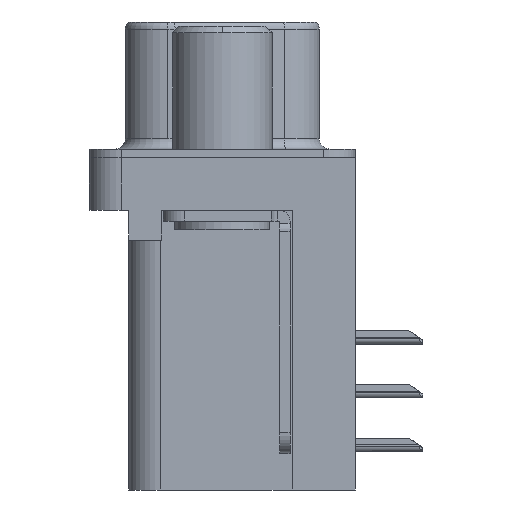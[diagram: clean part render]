
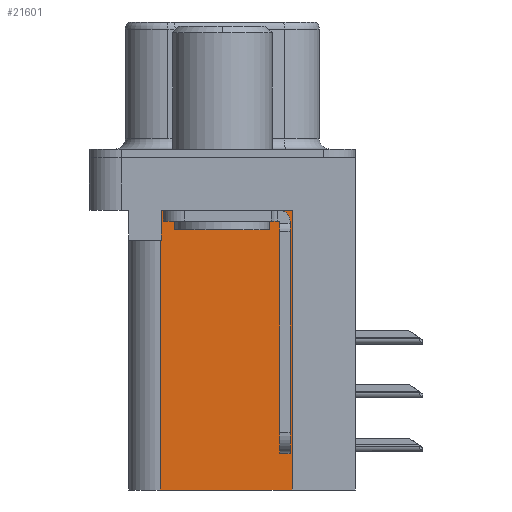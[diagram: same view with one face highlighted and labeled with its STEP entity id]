
A CAD part, left-side view. The second image highlights one B-rep face of the part: STEP entity #21601.
In plain terms, the highlighted planar face has unit normal (-1, 0, 0).
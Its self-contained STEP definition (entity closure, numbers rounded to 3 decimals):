
#147 = LINE ( 'NONE', #256, #7849 ) ;
#256 = CARTESIAN_POINT ( 'NONE',  ( 3.79, -3.295, -2.5 ) ) ;
#668 = EDGE_CURVE ( 'NONE', #18045, #21970, #11261, .T. ) ;
#2689 = VECTOR ( 'NONE', #6367, 1000. ) ;
#3335 = CARTESIAN_POINT ( 'NONE',  ( 3.79, -3.295, -2.5 ) ) ;
#3836 = EDGE_CURVE ( 'NONE', #22131, #28776, #23106, .T. ) ;
#4481 = PLANE ( 'NONE',  #26786 ) ;
#4844 = ORIENTED_EDGE ( 'NONE', *, *, #17191, .T. ) ;
#4858 = VECTOR ( 'NONE', #14583, 1000. ) ;
#5062 = ORIENTED_EDGE ( 'NONE', *, *, #3836, .T. ) ;
#6367 = DIRECTION ( 'NONE',  ( 0., 0., -1. ) ) ;
#6426 = LINE ( 'NONE', #26292, #26932 ) ;
#6596 = EDGE_LOOP ( 'NONE', ( #20667, #27789, #5062, #28978, #11658, #4844 ) ) ;
#7565 = CARTESIAN_POINT ( 'NONE',  ( 3.79, 0., -3.9 ) ) ;
#7719 = VECTOR ( 'NONE', #26728, 1000. ) ;
#7849 = VECTOR ( 'NONE', #13999, 1000. ) ;
#11261 = LINE ( 'NONE', #20682, #4858 ) ;
#11658 = ORIENTED_EDGE ( 'NONE', *, *, #668, .F. ) ;
#12693 = VERTEX_POINT ( 'NONE', #3335 ) ;
#13999 = DIRECTION ( 'NONE',  ( 0., 1., 0. ) ) ;
#14583 = DIRECTION ( 'NONE',  ( 0., 1., 0. ) ) ;
#16010 = CARTESIAN_POINT ( 'NONE',  ( 3.79, 2.925, -15.7 ) ) ;
#17191 = EDGE_CURVE ( 'NONE', #18045, #12693, #6426, .T. ) ;
#17584 = CARTESIAN_POINT ( 'NONE',  ( 3.79, -3.295, -15.7 ) ) ;
#18045 = VERTEX_POINT ( 'NONE', #17584 ) ;
#18079 = DIRECTION ( 'NONE',  ( 0., 1., 0. ) ) ;
#18216 = DIRECTION ( 'NONE',  ( 0., 0., 1. ) ) ;
#18395 = CARTESIAN_POINT ( 'NONE',  ( 3.79, 2.895, -2.5 ) ) ;
#18473 = EDGE_CURVE ( 'NONE', #21970, #28776, #21713, .T. ) ;
#20667 = ORIENTED_EDGE ( 'NONE', *, *, #28998, .T. ) ;
#20682 = CARTESIAN_POINT ( 'NONE',  ( 3.79, -3.295, -15.7 ) ) ;
#21601 = ADVANCED_FACE ( 'NONE', ( #33226 ), #4481, .F. ) ;
#21713 = LINE ( 'NONE', #16010, #7719 ) ;
#21970 = VERTEX_POINT ( 'NONE', #33004 ) ;
#22131 = VERTEX_POINT ( 'NONE', #33439 ) ;
#22289 = CARTESIAN_POINT ( 'NONE',  ( 3.79, 2.895, -3.9 ) ) ;
#23106 = LINE ( 'NONE', #7565, #29615 ) ;
#23205 = CARTESIAN_POINT ( 'NONE',  ( 3.79, -3.295, -15.7 ) ) ;
#25995 = DIRECTION ( 'NONE',  ( 0., 0., -1. ) ) ;
#26219 = CARTESIAN_POINT ( 'NONE',  ( 3.79, 2.925, -3.9 ) ) ;
#26292 = CARTESIAN_POINT ( 'NONE',  ( 3.79, -3.295, -15.7 ) ) ;
#26728 = DIRECTION ( 'NONE',  ( 0., 0., 1. ) ) ;
#26786 = AXIS2_PLACEMENT_3D ( 'NONE', #23205, #34196, #25995 ) ;
#26932 = VECTOR ( 'NONE', #18216, 1000. ) ;
#27789 = ORIENTED_EDGE ( 'NONE', *, *, #34431, .T. ) ;
#28776 = VERTEX_POINT ( 'NONE', #26219 ) ;
#28978 = ORIENTED_EDGE ( 'NONE', *, *, #18473, .F. ) ;
#28998 = EDGE_CURVE ( 'NONE', #12693, #32843, #147, .T. ) ;
#29615 = VECTOR ( 'NONE', #18079, 1000. ) ;
#30685 = LINE ( 'NONE', #22289, #2689 ) ;
#32843 = VERTEX_POINT ( 'NONE', #18395 ) ;
#33004 = CARTESIAN_POINT ( 'NONE',  ( 3.79, 2.925, -15.7 ) ) ;
#33226 = FACE_OUTER_BOUND ( 'NONE', #6596, .T. ) ;
#33439 = CARTESIAN_POINT ( 'NONE',  ( 3.79, 2.895, -3.9 ) ) ;
#34196 = DIRECTION ( 'NONE',  ( 1., 0., 0. ) ) ;
#34431 = EDGE_CURVE ( 'NONE', #32843, #22131, #30685, .T. ) ;
